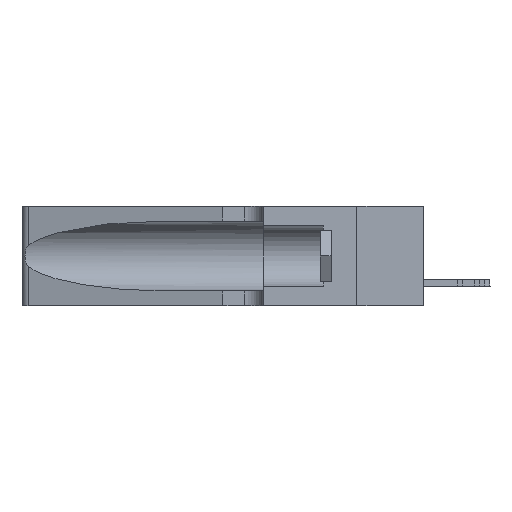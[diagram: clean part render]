
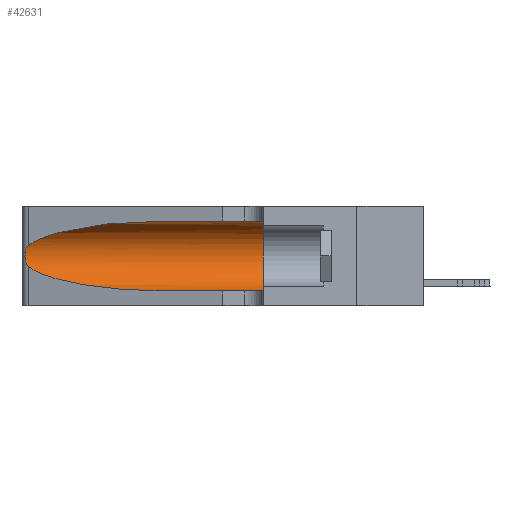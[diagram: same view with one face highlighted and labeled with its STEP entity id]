
A CAD part, left-side view. The second image highlights one B-rep face of the part: STEP entity #42631.
In plain terms, the highlighted cylindrical face has radius 3.308 mm (diameter 6.617 mm), a partial arc.
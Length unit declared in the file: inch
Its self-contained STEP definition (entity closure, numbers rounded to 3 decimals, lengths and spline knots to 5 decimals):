
#296 =( BOUNDED_CURVE ( )  B_SPLINE_CURVE ( 3, ( #30640, #16527, #5982, #19721 ),
 .UNSPECIFIED., .F., .F. ) 
 B_SPLINE_CURVE_WITH_KNOTS ( ( 4, 4 ),
 ( 1.5708, 2.84003 ),
 .UNSPECIFIED. ) 
 CURVE ( )  GEOMETRIC_REPRESENTATION_ITEM ( )  RATIONAL_B_SPLINE_CURVE ( ( 1., 0.87, 0.87, 1. ) ) 
 REPRESENTATION_ITEM ( '' )  );
#1522 = VECTOR ( 'NONE', #33945, 39.37008 ) ;
#2043 = CARTESIAN_POINT ( 'NONE',  ( 0.25487, 1.22718, 0.14631 ) ) ;
#2527 = DIRECTION ( 'NONE',  ( 0., 0., -1. ) ) ;
#5920 = CARTESIAN_POINT ( 'NONE',  ( 0.26017, 1.23833, 0.17102 ) ) ;
#5982 = CARTESIAN_POINT ( 'NONE',  ( 0.2373, 1.15595, 0.28018 ) ) ;
#6073 = CARTESIAN_POINT ( 'NONE',  ( 0.25487, 1.22718, 0.22369 ) ) ;
#7642 = CARTESIAN_POINT ( 'NONE',  ( 0.1305, 0.35, 0.185 ) ) ;
#9123 = CARTESIAN_POINT ( 'NONE',  ( 0.25854, 1.2359, 0.20912 ) ) ;
#9846 = CARTESIAN_POINT ( 'NONE',  ( 0.25487, 1.22718, 0.14631 ) ) ;
#10139 = ORIENTED_EDGE ( 'NONE', *, *, #34003, .F. ) ;
#10664 = ORIENTED_EDGE ( 'NONE', *, *, #39604, .T. ) ;
#11344 = EDGE_LOOP ( 'NONE', ( #30353, #23828, #11462, #10664, #10139, #42774 ) ) ;
#11462 = ORIENTED_EDGE ( 'NONE', *, *, #37192, .T. ) ;
#12780 = CARTESIAN_POINT ( 'NONE',  ( 0.26018, 1.23835, 0.19895 ) ) ;
#12925 = CARTESIAN_POINT ( 'NONE',  ( 0.1305, 0.35, 0.05475 ) ) ;
#13095 = CARTESIAN_POINT ( 'NONE',  ( 0.1305, 1.61858, 0.185 ) ) ;
#14641 =( BOUNDED_CURVE ( )  B_SPLINE_CURVE ( 3, ( #9846, #23909, #30960, #34464 ),
 .UNSPECIFIED., .F., .T. ) 
 B_SPLINE_CURVE_WITH_KNOTS ( ( 4, 4 ),
 ( 3.44316, 4.71239 ),
 .UNSPECIFIED. ) 
 CURVE ( )  GEOMETRIC_REPRESENTATION_ITEM ( )  RATIONAL_B_SPLINE_CURVE ( ( 1., 0.87, 0.87, 1. ) ) 
 REPRESENTATION_ITEM ( '' )  );
#16318 = LINE ( 'NONE', #29834, #1522 ) ;
#16527 = CARTESIAN_POINT ( 'NONE',  ( 0.18966, 0.96281, 0.31525 ) ) ;
#16628 = CARTESIAN_POINT ( 'NONE',  ( 0.26075, 1.23896, 0.19203 ) ) ;
#17142 = FACE_OUTER_BOUND ( 'NONE', #11344, .T. ) ;
#18934 = AXIS2_PLACEMENT_3D ( 'NONE', #13095, #37584, #2527 ) ;
#19721 = CARTESIAN_POINT ( 'NONE',  ( 0.25487, 1.22718, 0.22369 ) ) ;
#19942 = CARTESIAN_POINT ( 'NONE',  ( 0.1305, 0.72297, 0.31525 ) ) ;
#20263 = CARTESIAN_POINT ( 'NONE',  ( 0.25787, 1.23484, 0.2124 ) ) ;
#21383 = DIRECTION ( 'NONE',  ( 0., 0., 1. ) ) ;
#21844 = VERTEX_POINT ( 'NONE', #36131 ) ;
#22348 = CARTESIAN_POINT ( 'NONE',  ( 0.25487, 1.22718, 0.14631 ) ) ;
#23490 = CARTESIAN_POINT ( 'NONE',  ( 0.1305, 0.35, 0.31525 ) ) ;
#23828 = ORIENTED_EDGE ( 'NONE', *, *, #25007, .T. ) ;
#23909 = CARTESIAN_POINT ( 'NONE',  ( 0.2373, 1.15595, 0.08982 ) ) ;
#24295 = VECTOR ( 'NONE', #33997, 39.37008 ) ;
#25007 = EDGE_CURVE ( 'NONE', #21844, #34912, #41111, .T. ) ;
#26662 = EDGE_CURVE ( 'NONE', #36529, #31956, #16318, .T. ) ;
#26753 = CARTESIAN_POINT ( 'NONE',  ( 0.25856, 1.23593, 0.16098 ) ) ;
#26928 = CARTESIAN_POINT ( 'NONE',  ( 0.1305, 0.72297, 0.05475 ) ) ;
#27221 = CARTESIAN_POINT ( 'NONE',  ( 0.25639, 1.23186, 0.15144 ) ) ;
#29834 = CARTESIAN_POINT ( 'NONE',  ( 0.1305, 1.61858, 0.31525 ) ) ;
#30353 = ORIENTED_EDGE ( 'NONE', *, *, #41959, .T. ) ;
#30640 = CARTESIAN_POINT ( 'NONE',  ( 0.1305, 0.72297, 0.31525 ) ) ;
#30960 = CARTESIAN_POINT ( 'NONE',  ( 0.18966, 0.96281, 0.05475 ) ) ;
#31055 = VERTEX_POINT ( 'NONE', #12925 ) ;
#31408 = AXIS2_PLACEMENT_3D ( 'NONE', #7642, #39133, #21383 ) ;
#31931 = CYLINDRICAL_SURFACE ( 'NONE', #18934, 0.13025 ) ;
#31956 = VERTEX_POINT ( 'NONE', #23490 ) ;
#33912 = CARTESIAN_POINT ( 'NONE',  ( 0.25789, 1.23486, 0.15765 ) ) ;
#33945 = DIRECTION ( 'NONE',  ( 0., -1., 0. ) ) ;
#33997 = DIRECTION ( 'NONE',  ( 0., -1., 0. ) ) ;
#34003 = EDGE_CURVE ( 'NONE', #31956, #31055, #36603, .T. ) ;
#34225 = CARTESIAN_POINT ( 'NONE',  ( 0.25639, 1.23184, 0.21858 ) ) ;
#34464 = CARTESIAN_POINT ( 'NONE',  ( 0.1305, 0.72297, 0.05475 ) ) ;
#34912 = VERTEX_POINT ( 'NONE', #22348 ) ;
#35891 = VERTEX_POINT ( 'NONE', #26928 ) ;
#36131 = CARTESIAN_POINT ( 'NONE',  ( 0.25487, 1.22718, 0.22369 ) ) ;
#36529 = VERTEX_POINT ( 'NONE', #19942 ) ;
#36603 = CIRCLE ( 'NONE', #31408, 0.13025 ) ;
#37192 = EDGE_CURVE ( 'NONE', #34912, #35891, #14641, .T. ) ;
#37416 = LINE ( 'NONE', #41210, #24295 ) ;
#37577 = CARTESIAN_POINT ( 'NONE',  ( 0.25555, 1.22994, 0.2215 ) ) ;
#37584 = DIRECTION ( 'NONE',  ( 0., -1., 0. ) ) ;
#39133 = DIRECTION ( 'NONE',  ( 0., 1., 0. ) ) ;
#39604 = EDGE_CURVE ( 'NONE', #35891, #31055, #37416, .T. ) ;
#41111 = B_SPLINE_CURVE_WITH_KNOTS ( 'NONE', 3,
 ( #6073, #37577, #34225, #20263, #9123, #12780, #16628, #41118, #5920, #26753, #33912, #27221, #44814, #2043 ),
 .UNSPECIFIED., .F., .F.,
 ( 4, 2, 2, 2, 2, 2, 4 ),
 ( 0., 0.00027, 0.00053, 0.00107, 0.0016, 0.00187, 0.00214 ),
 .UNSPECIFIED. ) ;
#41118 = CARTESIAN_POINT ( 'NONE',  ( 0.26075, 1.23896, 0.178 ) ) ;
#41210 = CARTESIAN_POINT ( 'NONE',  ( 0.1305, 1.61858, 0.05475 ) ) ;
#41959 = EDGE_CURVE ( 'NONE', #36529, #21844, #296, .T. ) ;
#42631 = ADVANCED_FACE ( 'NONE', ( #17142 ), #31931, .F. ) ;
#42774 = ORIENTED_EDGE ( 'NONE', *, *, #26662, .F. ) ;
#44814 = CARTESIAN_POINT ( 'NONE',  ( 0.25555, 1.22993, 0.14849 ) ) ;
